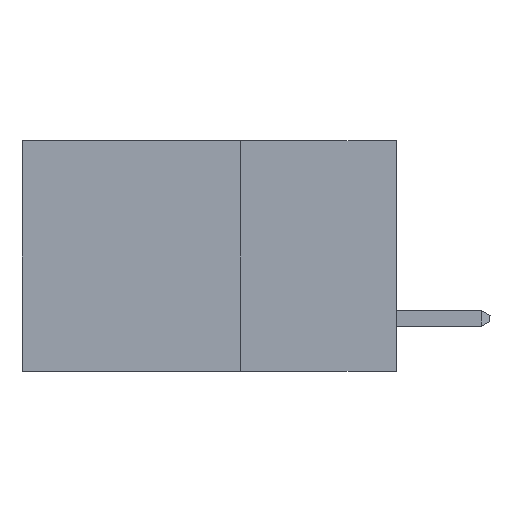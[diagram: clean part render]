
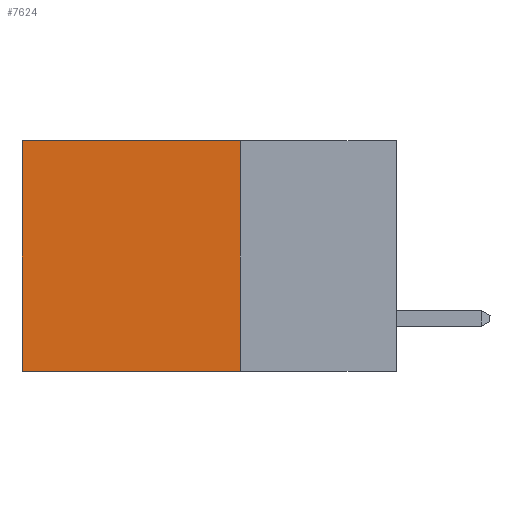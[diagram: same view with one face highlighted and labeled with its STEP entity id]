
A CAD part, left-side view. The second image highlights one B-rep face of the part: STEP entity #7624.
In plain terms, the highlighted planar face has unit normal (-1, 0, 0).
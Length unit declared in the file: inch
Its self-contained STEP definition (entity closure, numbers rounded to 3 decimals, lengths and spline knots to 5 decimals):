
#43 = DIRECTION ( 'NONE',  ( 0., 1., 0. ) ) ;
#191 = LINE ( 'NONE', #19594, #10476 ) ;
#1341 = VERTEX_POINT ( 'NONE', #18251 ) ;
#3033 = CARTESIAN_POINT ( 'NONE',  ( 0.2615, 0.25, 0. ) ) ;
#3189 = PLANE ( 'NONE',  #18602 ) ;
#3447 = EDGE_LOOP ( 'NONE', ( #6608, #11922, #4677, #22130 ) ) ;
#3786 = VERTEX_POINT ( 'NONE', #3033 ) ;
#3793 = VECTOR ( 'NONE', #10599, 39.37008 ) ;
#4130 = LINE ( 'NONE', #21624, #19169 ) ;
#4677 = ORIENTED_EDGE ( 'NONE', *, *, #14984, .F. ) ;
#4860 = DIRECTION ( 'NONE',  ( 1., 0., 0. ) ) ;
#5252 = VERTEX_POINT ( 'NONE', #7643 ) ;
#5457 = CARTESIAN_POINT ( 'NONE',  ( 0.2615, 0.25, -0.37 ) ) ;
#5673 = VERTEX_POINT ( 'NONE', #5457 ) ;
#6050 = DIRECTION ( 'NONE',  ( 0., 0., -1. ) ) ;
#6090 = DIRECTION ( 'NONE',  ( 0., 1., 0. ) ) ;
#6608 = ORIENTED_EDGE ( 'NONE', *, *, #13533, .T. ) ;
#7624 = ADVANCED_FACE ( 'NONE', ( #20668 ), #3189, .F. ) ;
#7643 = CARTESIAN_POINT ( 'NONE',  ( 0.2615, 0.6, -0.37 ) ) ;
#7706 = CARTESIAN_POINT ( 'NONE',  ( 0.2615, 0.6, -0.37 ) ) ;
#7895 = VECTOR ( 'NONE', #6050, 39.37008 ) ;
#8817 = CARTESIAN_POINT ( 'NONE',  ( 0.2615, 0.25, -0.37 ) ) ;
#10073 = EDGE_CURVE ( 'NONE', #5673, #5252, #4130, .T. ) ;
#10476 = VECTOR ( 'NONE', #6090, 39.37008 ) ;
#10599 = DIRECTION ( 'NONE',  ( 0., 0., -1. ) ) ;
#11922 = ORIENTED_EDGE ( 'NONE', *, *, #10073, .F. ) ;
#12261 = CARTESIAN_POINT ( 'NONE',  ( 0.2615, 0.25, -0.37 ) ) ;
#12365 = DIRECTION ( 'NONE',  ( 0., 0., -1. ) ) ;
#13533 = EDGE_CURVE ( 'NONE', #1341, #5252, #15841, .T. ) ;
#14984 = EDGE_CURVE ( 'NONE', #3786, #5673, #15717, .T. ) ;
#15717 = LINE ( 'NONE', #12261, #3793 ) ;
#15841 = LINE ( 'NONE', #7706, #7895 ) ;
#18251 = CARTESIAN_POINT ( 'NONE',  ( 0.2615, 0.6, 0. ) ) ;
#18602 = AXIS2_PLACEMENT_3D ( 'NONE', #8817, #4860, #12365 ) ;
#19169 = VECTOR ( 'NONE', #43, 39.37008 ) ;
#19594 = CARTESIAN_POINT ( 'NONE',  ( 0.2615, 0.25, 0. ) ) ;
#20223 = EDGE_CURVE ( 'NONE', #3786, #1341, #191, .T. ) ;
#20668 = FACE_OUTER_BOUND ( 'NONE', #3447, .T. ) ;
#21624 = CARTESIAN_POINT ( 'NONE',  ( 0.2615, 0.25, -0.37 ) ) ;
#22130 = ORIENTED_EDGE ( 'NONE', *, *, #20223, .T. ) ;
